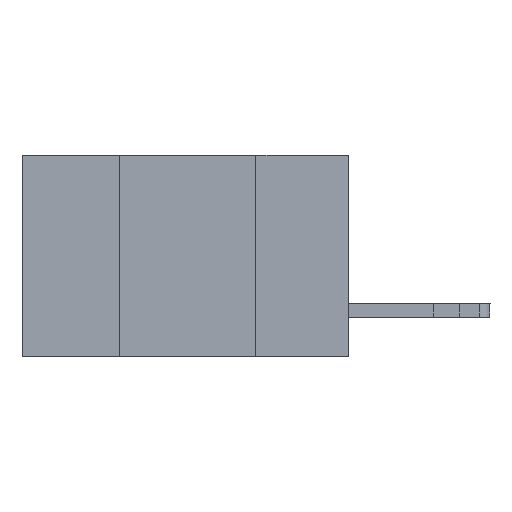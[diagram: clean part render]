
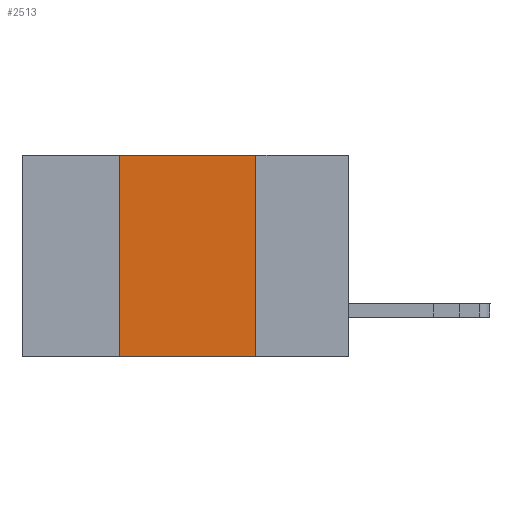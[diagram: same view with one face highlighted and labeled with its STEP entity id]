
A CAD part, left-side view. The second image highlights one B-rep face of the part: STEP entity #2513.
In plain terms, the highlighted planar face has unit normal (-1, 0, 0).
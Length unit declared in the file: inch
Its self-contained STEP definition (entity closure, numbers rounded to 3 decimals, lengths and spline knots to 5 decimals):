
#4 = DIRECTION ( 'NONE',  ( 0., -1., 0. ) ) ;
#232 = VERTEX_POINT ( 'NONE', #7408 ) ;
#367 = AXIS2_PLACEMENT_3D ( 'NONE', #4766, #20063, #13098 ) ;
#521 = VECTOR ( 'NONE', #18711, 39.37008 ) ;
#895 = CARTESIAN_POINT ( 'NONE',  ( 0., 0.6, -0.37 ) ) ;
#974 = PLANE ( 'NONE',  #367 ) ;
#2513 = ADVANCED_FACE ( 'NONE', ( #9656 ), #974, .F. ) ;
#4244 = CARTESIAN_POINT ( 'NONE',  ( 0., 0.42, -0.37 ) ) ;
#4766 = CARTESIAN_POINT ( 'NONE',  ( 0., 0.6, 0. ) ) ;
#4804 = VECTOR ( 'NONE', #20457, 39.37008 ) ;
#5895 = ORIENTED_EDGE ( 'NONE', *, *, #18723, .T. ) ;
#6742 = ORIENTED_EDGE ( 'NONE', *, *, #12212, .F. ) ;
#7408 = CARTESIAN_POINT ( 'NONE',  ( 0., 0.17, -0.37 ) ) ;
#8453 = LINE ( 'NONE', #15240, #12197 ) ;
#8653 = VERTEX_POINT ( 'NONE', #4244 ) ;
#9656 = FACE_OUTER_BOUND ( 'NONE', #20253, .T. ) ;
#10051 = LINE ( 'NONE', #21894, #4804 ) ;
#12197 = VECTOR ( 'NONE', #4, 39.37008 ) ;
#12212 = EDGE_CURVE ( 'NONE', #16830, #19850, #8453, .T. ) ;
#12479 = CARTESIAN_POINT ( 'NONE',  ( 0., 0.17, 0. ) ) ;
#13098 = DIRECTION ( 'NONE',  ( 0., 0., -1. ) ) ;
#13739 = EDGE_CURVE ( 'NONE', #8653, #16830, #15218, .T. ) ;
#13892 = CARTESIAN_POINT ( 'NONE',  ( 0., 0.42, 0. ) ) ;
#14369 = LINE ( 'NONE', #895, #16976 ) ;
#14645 = EDGE_CURVE ( 'NONE', #19850, #232, #10051, .T. ) ;
#15218 = LINE ( 'NONE', #13892, #521 ) ;
#15240 = CARTESIAN_POINT ( 'NONE',  ( 0., 0.6, 0. ) ) ;
#15948 = CARTESIAN_POINT ( 'NONE',  ( 0., 0.42, 0. ) ) ;
#16250 = DIRECTION ( 'NONE',  ( 0., -1., 0. ) ) ;
#16830 = VERTEX_POINT ( 'NONE', #15948 ) ;
#16976 = VECTOR ( 'NONE', #16250, 39.37008 ) ;
#17517 = ORIENTED_EDGE ( 'NONE', *, *, #14645, .F. ) ;
#18711 = DIRECTION ( 'NONE',  ( 0., 0., 1. ) ) ;
#18723 = EDGE_CURVE ( 'NONE', #8653, #232, #14369, .T. ) ;
#19850 = VERTEX_POINT ( 'NONE', #12479 ) ;
#20063 = DIRECTION ( 'NONE',  ( 1., 0., 0. ) ) ;
#20253 = EDGE_LOOP ( 'NONE', ( #17517, #6742, #20328, #5895 ) ) ;
#20328 = ORIENTED_EDGE ( 'NONE', *, *, #13739, .F. ) ;
#20457 = DIRECTION ( 'NONE',  ( 0., 0., -1. ) ) ;
#21894 = CARTESIAN_POINT ( 'NONE',  ( 0., 0.17, 0. ) ) ;
